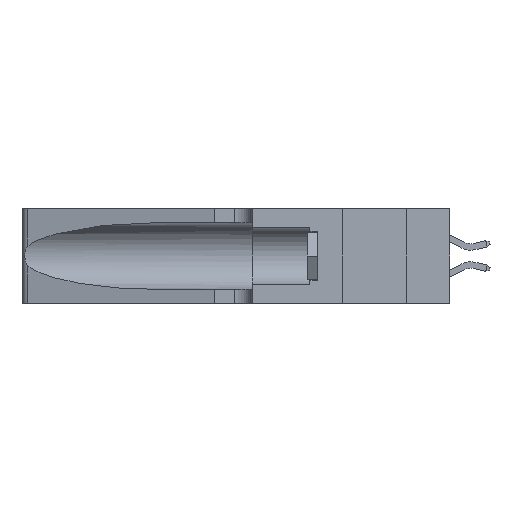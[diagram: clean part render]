
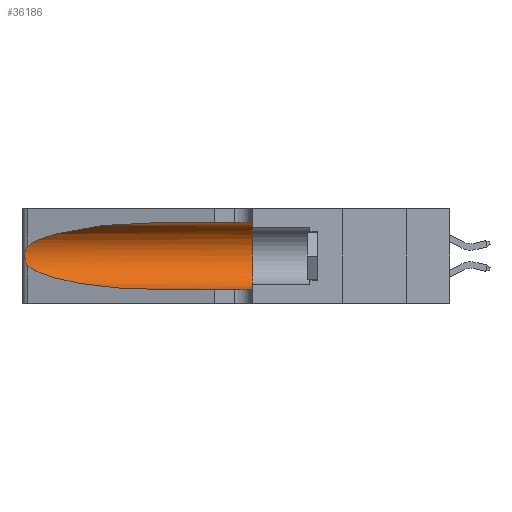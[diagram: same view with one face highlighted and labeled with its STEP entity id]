
A CAD part, left-side view. The second image highlights one B-rep face of the part: STEP entity #36186.
In plain terms, the highlighted cylindrical face has radius 3.308 mm (diameter 6.617 mm), a partial arc.
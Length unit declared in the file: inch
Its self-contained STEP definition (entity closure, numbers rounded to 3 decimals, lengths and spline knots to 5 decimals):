
#1146 = CARTESIAN_POINT ( 'NONE',  ( 0.25487, 1.22718, 0.22369 ) ) ;
#1541 = DIRECTION ( 'NONE',  ( 0., 0., -1. ) ) ;
#1654 = CARTESIAN_POINT ( 'NONE',  ( 0.25639, 1.23184, 0.21858 ) ) ;
#2234 = DIRECTION ( 'NONE',  ( 0., 0., 1. ) ) ;
#2498 = EDGE_CURVE ( 'NONE', #23901, #20311, #21192, .T. ) ;
#2526 = CARTESIAN_POINT ( 'NONE',  ( 0.1305, 0.72297, 0.31525 ) ) ;
#2833 = EDGE_CURVE ( 'NONE', #24999, #23901, #20730, .T. ) ;
#2898 = ORIENTED_EDGE ( 'NONE', *, *, #29245, .T. ) ;
#3993 = EDGE_CURVE ( 'NONE', #24999, #25117, #11116, .T. ) ;
#4681 = CARTESIAN_POINT ( 'NONE',  ( 0.25854, 1.2359, 0.20912 ) ) ;
#5641 = CARTESIAN_POINT ( 'NONE',  ( 0.1305, 0.72297, 0.05475 ) ) ;
#6139 =( BOUNDED_CURVE ( )  B_SPLINE_CURVE ( 3, ( #27114, #30041, #12429, #32914 ),
 .UNSPECIFIED., .F., .F. ) 
 B_SPLINE_CURVE_WITH_KNOTS ( ( 4, 4 ),
 ( 3.44316, 4.71239 ),
 .UNSPECIFIED. ) 
 CURVE ( )  GEOMETRIC_REPRESENTATION_ITEM ( )  RATIONAL_B_SPLINE_CURVE ( ( 1., 0.87, 0.87, 1. ) ) 
 REPRESENTATION_ITEM ( '' )  );
#6640 = CARTESIAN_POINT ( 'NONE',  ( 0.1305, 0.35, 0.05475 ) ) ;
#7708 = CARTESIAN_POINT ( 'NONE',  ( 0.26075, 1.23896, 0.19203 ) ) ;
#8038 = VECTOR ( 'NONE', #11431, 39.37008 ) ;
#8573 = CARTESIAN_POINT ( 'NONE',  ( 0.2373, 1.15595, 0.28018 ) ) ;
#10653 = B_SPLINE_CURVE_WITH_KNOTS ( 'NONE', 3,
 ( #31087, #16487, #1654, #22418, #4681, #25374, #7708, #28303, #10678, #31205, #13630, #34096, #16624, #36995 ),
 .UNSPECIFIED., .F., .F.,
 ( 4, 2, 2, 2, 2, 2, 4 ),
 ( 0., 0.00027, 0.00053, 0.00107, 0.0016, 0.00187, 0.00214 ),
 .UNSPECIFIED. ) ;
#10678 = CARTESIAN_POINT ( 'NONE',  ( 0.26017, 1.23833, 0.17102 ) ) ;
#11116 =( BOUNDED_CURVE ( )  B_SPLINE_CURVE ( 3, ( #2526, #29150, #8573, #14480 ),
 .UNSPECIFIED., .F., .F. ) 
 B_SPLINE_CURVE_WITH_KNOTS ( ( 4, 4 ),
 ( 1.5708, 2.84003 ),
 .UNSPECIFIED. ) 
 CURVE ( )  GEOMETRIC_REPRESENTATION_ITEM ( )  RATIONAL_B_SPLINE_CURVE ( ( 1., 0.87, 0.87, 1. ) ) 
 REPRESENTATION_ITEM ( '' )  );
#11431 = DIRECTION ( 'NONE',  ( 0., -1., 0. ) ) ;
#12429 = CARTESIAN_POINT ( 'NONE',  ( 0.18966, 0.96281, 0.05475 ) ) ;
#13630 = CARTESIAN_POINT ( 'NONE',  ( 0.25789, 1.23486, 0.15765 ) ) ;
#14078 = AXIS2_PLACEMENT_3D ( 'NONE', #37422, #20051, #2234 ) ;
#14480 = CARTESIAN_POINT ( 'NONE',  ( 0.25487, 1.22718, 0.22369 ) ) ;
#15446 = CARTESIAN_POINT ( 'NONE',  ( 0.1305, 0.72297, 0.31525 ) ) ;
#16368 = DIRECTION ( 'NONE',  ( 0., -1., 0. ) ) ;
#16487 = CARTESIAN_POINT ( 'NONE',  ( 0.25555, 1.22994, 0.2215 ) ) ;
#16624 = CARTESIAN_POINT ( 'NONE',  ( 0.25555, 1.22993, 0.14849 ) ) ;
#17023 = VECTOR ( 'NONE', #21424, 39.37008 ) ;
#17906 = ORIENTED_EDGE ( 'NONE', *, *, #23320, .T. ) ;
#18300 = FACE_OUTER_BOUND ( 'NONE', #23338, .T. ) ;
#18574 = EDGE_CURVE ( 'NONE', #26887, #27106, #6139, .T. ) ;
#20051 = DIRECTION ( 'NONE',  ( 0., 1., 0. ) ) ;
#20311 = VERTEX_POINT ( 'NONE', #6640 ) ;
#20730 = LINE ( 'NONE', #24259, #17023 ) ;
#21192 = CIRCLE ( 'NONE', #14078, 0.13025 ) ;
#21424 = DIRECTION ( 'NONE',  ( 0., -1., 0. ) ) ;
#22418 = CARTESIAN_POINT ( 'NONE',  ( 0.25787, 1.23484, 0.2124 ) ) ;
#23320 = EDGE_CURVE ( 'NONE', #25117, #26887, #10653, .T. ) ;
#23338 = EDGE_LOOP ( 'NONE', ( #34540, #17906, #23700, #2898, #34145, #37156 ) ) ;
#23700 = ORIENTED_EDGE ( 'NONE', *, *, #18574, .T. ) ;
#23901 = VERTEX_POINT ( 'NONE', #36441 ) ;
#24259 = CARTESIAN_POINT ( 'NONE',  ( 0.1305, 1.61858, 0.31525 ) ) ;
#24667 = LINE ( 'NONE', #34846, #8038 ) ;
#24999 = VERTEX_POINT ( 'NONE', #15446 ) ;
#25095 = AXIS2_PLACEMENT_3D ( 'NONE', #36743, #16368, #1541 ) ;
#25117 = VERTEX_POINT ( 'NONE', #1146 ) ;
#25374 = CARTESIAN_POINT ( 'NONE',  ( 0.26018, 1.23835, 0.19895 ) ) ;
#26887 = VERTEX_POINT ( 'NONE', #28212 ) ;
#27106 = VERTEX_POINT ( 'NONE', #5641 ) ;
#27114 = CARTESIAN_POINT ( 'NONE',  ( 0.25487, 1.22718, 0.14631 ) ) ;
#28212 = CARTESIAN_POINT ( 'NONE',  ( 0.25487, 1.22718, 0.14631 ) ) ;
#28303 = CARTESIAN_POINT ( 'NONE',  ( 0.26075, 1.23896, 0.178 ) ) ;
#29150 = CARTESIAN_POINT ( 'NONE',  ( 0.18966, 0.96281, 0.31525 ) ) ;
#29245 = EDGE_CURVE ( 'NONE', #27106, #20311, #24667, .T. ) ;
#30041 = CARTESIAN_POINT ( 'NONE',  ( 0.2373, 1.15595, 0.08982 ) ) ;
#31087 = CARTESIAN_POINT ( 'NONE',  ( 0.25487, 1.22718, 0.22369 ) ) ;
#31205 = CARTESIAN_POINT ( 'NONE',  ( 0.25856, 1.23593, 0.16098 ) ) ;
#32859 = CYLINDRICAL_SURFACE ( 'NONE', #25095, 0.13025 ) ;
#32914 = CARTESIAN_POINT ( 'NONE',  ( 0.1305, 0.72297, 0.05475 ) ) ;
#34096 = CARTESIAN_POINT ( 'NONE',  ( 0.25639, 1.23186, 0.15144 ) ) ;
#34145 = ORIENTED_EDGE ( 'NONE', *, *, #2498, .F. ) ;
#34540 = ORIENTED_EDGE ( 'NONE', *, *, #3993, .T. ) ;
#34846 = CARTESIAN_POINT ( 'NONE',  ( 0.1305, 1.61858, 0.05475 ) ) ;
#36186 = ADVANCED_FACE ( 'NONE', ( #18300 ), #32859, .F. ) ;
#36441 = CARTESIAN_POINT ( 'NONE',  ( 0.1305, 0.35, 0.31525 ) ) ;
#36743 = CARTESIAN_POINT ( 'NONE',  ( 0.1305, 1.61858, 0.185 ) ) ;
#36995 = CARTESIAN_POINT ( 'NONE',  ( 0.25487, 1.22718, 0.14631 ) ) ;
#37156 = ORIENTED_EDGE ( 'NONE', *, *, #2833, .F. ) ;
#37422 = CARTESIAN_POINT ( 'NONE',  ( 0.1305, 0.35, 0.185 ) ) ;
